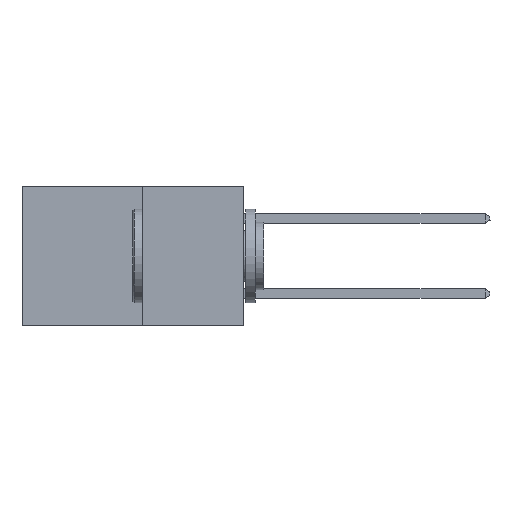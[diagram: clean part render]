
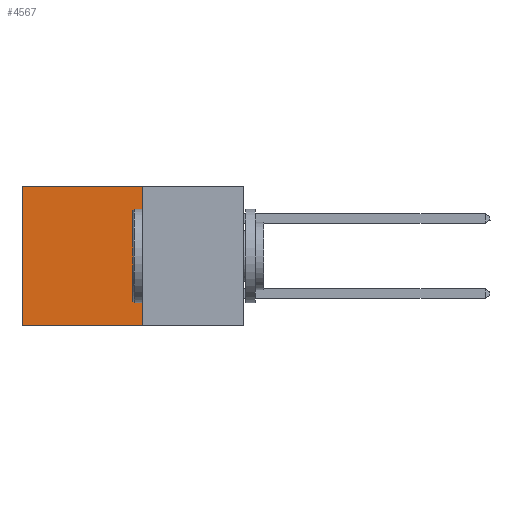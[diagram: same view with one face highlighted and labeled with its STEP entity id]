
A CAD part, left-side view. The second image highlights one B-rep face of the part: STEP entity #4567.
In plain terms, the highlighted planar face has unit normal (-1, 0, 0).
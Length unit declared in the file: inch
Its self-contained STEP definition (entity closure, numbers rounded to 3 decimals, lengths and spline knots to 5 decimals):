
#974 = LINE ( 'NONE', #7597, #6013 ) ;
#1803 = VECTOR ( 'NONE', #12510, 39.37008 ) ;
#2119 = DIRECTION ( 'NONE',  ( 0., 1., 0. ) ) ;
#2389 = AXIS2_PLACEMENT_3D ( 'NONE', #11774, #11301, #11276 ) ;
#2442 = ORIENTED_EDGE ( 'NONE', *, *, #10605, .T. ) ;
#3001 = ORIENTED_EDGE ( 'NONE', *, *, #9382, .T. ) ;
#3042 = ORIENTED_EDGE ( 'NONE', *, *, #4386, .F. ) ;
#3141 = VERTEX_POINT ( 'NONE', #4102 ) ;
#3678 = CARTESIAN_POINT ( 'NONE',  ( 0.277, 0.59, 0. ) ) ;
#4102 = CARTESIAN_POINT ( 'NONE',  ( 0.277, 0.27, 0. ) ) ;
#4386 = EDGE_CURVE ( 'NONE', #3141, #4440, #974, .T. ) ;
#4433 = CARTESIAN_POINT ( 'NONE',  ( 0.277, 0.27, -0.37 ) ) ;
#4440 = VERTEX_POINT ( 'NONE', #4433 ) ;
#4567 = ADVANCED_FACE ( 'NONE', ( #6179 ), #11370, .F. ) ;
#4623 = LINE ( 'NONE', #11514, #1803 ) ;
#5292 = EDGE_LOOP ( 'NONE', ( #3001, #12179, #3042, #2442 ) ) ;
#6013 = VECTOR ( 'NONE', #8128, 39.37008 ) ;
#6179 = FACE_OUTER_BOUND ( 'NONE', #5292, .T. ) ;
#6692 = EDGE_CURVE ( 'NONE', #4440, #10491, #9017, .T. ) ;
#7597 = CARTESIAN_POINT ( 'NONE',  ( 0.277, 0.27, -0.37 ) ) ;
#8128 = DIRECTION ( 'NONE',  ( 0., 0., -1. ) ) ;
#8334 = CARTESIAN_POINT ( 'NONE',  ( 0.277, 0.59, -0.37 ) ) ;
#9017 = LINE ( 'NONE', #12520, #11195 ) ;
#9382 = EDGE_CURVE ( 'NONE', #10920, #10491, #4623, .T. ) ;
#9484 = VECTOR ( 'NONE', #2119, 39.37008 ) ;
#9775 = LINE ( 'NONE', #10373, #9484 ) ;
#10373 = CARTESIAN_POINT ( 'NONE',  ( 0.277, 0.27, 0. ) ) ;
#10491 = VERTEX_POINT ( 'NONE', #8334 ) ;
#10605 = EDGE_CURVE ( 'NONE', #3141, #10920, #9775, .T. ) ;
#10920 = VERTEX_POINT ( 'NONE', #3678 ) ;
#11195 = VECTOR ( 'NONE', #12309, 39.37008 ) ;
#11276 = DIRECTION ( 'NONE',  ( 0., 0., -1. ) ) ;
#11301 = DIRECTION ( 'NONE',  ( 1., 0., 0. ) ) ;
#11370 = PLANE ( 'NONE',  #2389 ) ;
#11514 = CARTESIAN_POINT ( 'NONE',  ( 0.277, 0.59, -0.37 ) ) ;
#11774 = CARTESIAN_POINT ( 'NONE',  ( 0.277, 0.27, -0.37 ) ) ;
#12179 = ORIENTED_EDGE ( 'NONE', *, *, #6692, .F. ) ;
#12309 = DIRECTION ( 'NONE',  ( 0., 1., 0. ) ) ;
#12510 = DIRECTION ( 'NONE',  ( 0., 0., -1. ) ) ;
#12520 = CARTESIAN_POINT ( 'NONE',  ( 0.277, 0.27, -0.37 ) ) ;
